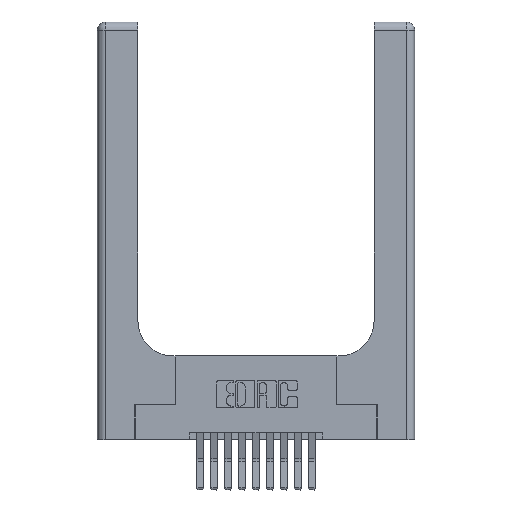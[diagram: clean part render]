
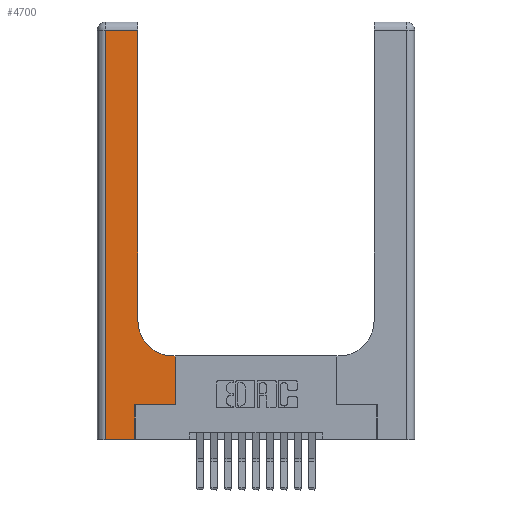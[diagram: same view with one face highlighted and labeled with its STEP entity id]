
A CAD part, top view. The second image highlights one B-rep face of the part: STEP entity #4700.
In plain terms, the highlighted planar face has unit normal (0, 0, 1).
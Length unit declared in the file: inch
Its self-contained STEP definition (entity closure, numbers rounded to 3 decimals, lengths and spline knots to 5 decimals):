
#72 = LINE ( 'NONE', #14565, #12407 ) ;
#222 = EDGE_CURVE ( 'NONE', #7299, #13981, #5925, .T. ) ;
#307 = DIRECTION ( 'NONE',  ( 0., -1., 0. ) ) ;
#822 = CARTESIAN_POINT ( 'NONE',  ( 0., 3., 0.37 ) ) ;
#990 = CARTESIAN_POINT ( 'NONE',  ( 0.5415, 0.85, 0.37 ) ) ;
#1524 = CARTESIAN_POINT ( 'NONE',  ( 0.2915, 3., 0.37 ) ) ;
#1644 = FACE_OUTER_BOUND ( 'NONE', #4326, .T. ) ;
#2067 = VECTOR ( 'NONE', #12881, 39.37008 ) ;
#2114 = DIRECTION ( 'NONE',  ( 0., 0., -1. ) ) ;
#2183 = DIRECTION ( 'NONE',  ( 1., 0., 0. ) ) ;
#2291 = VECTOR ( 'NONE', #4145, 39.37008 ) ;
#2648 = CARTESIAN_POINT ( 'NONE',  ( 0.269, 0.25, 0.37 ) ) ;
#3165 = VECTOR ( 'NONE', #307, 39.37008 ) ;
#3362 = DIRECTION ( 'NONE',  ( 0., 0., -1. ) ) ;
#3465 = EDGE_CURVE ( 'NONE', #14264, #10648, #11820, .T. ) ;
#3478 = PLANE ( 'NONE',  #10093 ) ;
#3799 = LINE ( 'NONE', #9825, #3165 ) ;
#3899 = LINE ( 'NONE', #6429, #2067 ) ;
#4033 = LINE ( 'NONE', #15352, #6666 ) ;
#4145 = DIRECTION ( 'NONE',  ( 0., 1., 0. ) ) ;
#4220 = CARTESIAN_POINT ( 'NONE',  ( 0.5415, 0.6, 0.37 ) ) ;
#4270 = CARTESIAN_POINT ( 'NONE',  ( 0.5585, 0.25, 0.37 ) ) ;
#4326 = EDGE_LOOP ( 'NONE', ( #11768, #13753, #9797, #5466, #5655, #13110, #4332, #12403, #4634 ) ) ;
#4332 = ORIENTED_EDGE ( 'NONE', *, *, #6078, .T. ) ;
#4634 = ORIENTED_EDGE ( 'NONE', *, *, #4713, .T. ) ;
#4700 = ADVANCED_FACE ( 'NONE', ( #1644 ), #3478, .F. ) ;
#4713 = EDGE_CURVE ( 'NONE', #5835, #7299, #9153, .T. ) ;
#4761 = VERTEX_POINT ( 'NONE', #6194 ) ;
#4928 = VERTEX_POINT ( 'NONE', #14402 ) ;
#5466 = ORIENTED_EDGE ( 'NONE', *, *, #7401, .T. ) ;
#5625 = LINE ( 'NONE', #4270, #6683 ) ;
#5655 = ORIENTED_EDGE ( 'NONE', *, *, #11003, .T. ) ;
#5835 = VERTEX_POINT ( 'NONE', #4220 ) ;
#5925 = LINE ( 'NONE', #1524, #2291 ) ;
#6078 = EDGE_CURVE ( 'NONE', #10648, #4761, #5625, .T. ) ;
#6194 = CARTESIAN_POINT ( 'NONE',  ( 0.5585, 0.6, 0.37 ) ) ;
#6277 = EDGE_CURVE ( 'NONE', #4761, #5835, #4033, .T. ) ;
#6429 = CARTESIAN_POINT ( 'NONE',  ( 0., 2.94, 0.37 ) ) ;
#6666 = VECTOR ( 'NONE', #11762, 39.37008 ) ;
#6683 = VECTOR ( 'NONE', #10739, 39.37008 ) ;
#7299 = VERTEX_POINT ( 'NONE', #11788 ) ;
#7401 = EDGE_CURVE ( 'NONE', #13030, #4928, #72, .T. ) ;
#7614 = LINE ( 'NONE', #12504, #13249 ) ;
#7795 = CARTESIAN_POINT ( 'NONE',  ( 0.06, 0., 0.37 ) ) ;
#8512 = CARTESIAN_POINT ( 'NONE',  ( 0.06, 2.94, 0.37 ) ) ;
#9153 = CIRCLE ( 'NONE', #11802, 0.25 ) ;
#9394 = VECTOR ( 'NONE', #14858, 39.37008 ) ;
#9561 = EDGE_CURVE ( 'NONE', #11232, #13030, #3799, .T. ) ;
#9797 = ORIENTED_EDGE ( 'NONE', *, *, #9561, .T. ) ;
#9825 = CARTESIAN_POINT ( 'NONE',  ( 0.06, 3., 0.37 ) ) ;
#10093 = AXIS2_PLACEMENT_3D ( 'NONE', #822, #3362, #15098 ) ;
#10648 = VERTEX_POINT ( 'NONE', #13576 ) ;
#10739 = DIRECTION ( 'NONE',  ( 0., 1., 0. ) ) ;
#10819 = CARTESIAN_POINT ( 'NONE',  ( 0.2915, 2.94, 0.37 ) ) ;
#11003 = EDGE_CURVE ( 'NONE', #4928, #14264, #7614, .T. ) ;
#11232 = VERTEX_POINT ( 'NONE', #8512 ) ;
#11762 = DIRECTION ( 'NONE',  ( -1., 0., 0. ) ) ;
#11768 = ORIENTED_EDGE ( 'NONE', *, *, #222, .T. ) ;
#11788 = CARTESIAN_POINT ( 'NONE',  ( 0.2915, 0.85, 0.37 ) ) ;
#11802 = AXIS2_PLACEMENT_3D ( 'NONE', #990, #2114, #2183 ) ;
#11820 = LINE ( 'NONE', #14799, #9394 ) ;
#12063 = DIRECTION ( 'NONE',  ( 1., 0., 0. ) ) ;
#12394 = DIRECTION ( 'NONE',  ( 0., 1., 0. ) ) ;
#12403 = ORIENTED_EDGE ( 'NONE', *, *, #6277, .T. ) ;
#12407 = VECTOR ( 'NONE', #12063, 39.37008 ) ;
#12504 = CARTESIAN_POINT ( 'NONE',  ( 0.269, 0., 0.37 ) ) ;
#12881 = DIRECTION ( 'NONE',  ( -1., 0., 0. ) ) ;
#13030 = VERTEX_POINT ( 'NONE', #7795 ) ;
#13110 = ORIENTED_EDGE ( 'NONE', *, *, #3465, .T. ) ;
#13249 = VECTOR ( 'NONE', #12394, 39.37008 ) ;
#13576 = CARTESIAN_POINT ( 'NONE',  ( 0.5585, 0.25, 0.37 ) ) ;
#13753 = ORIENTED_EDGE ( 'NONE', *, *, #15255, .T. ) ;
#13981 = VERTEX_POINT ( 'NONE', #10819 ) ;
#14264 = VERTEX_POINT ( 'NONE', #2648 ) ;
#14402 = CARTESIAN_POINT ( 'NONE',  ( 0.269, 0., 0.37 ) ) ;
#14565 = CARTESIAN_POINT ( 'NONE',  ( 0., 0., 0.37 ) ) ;
#14799 = CARTESIAN_POINT ( 'NONE',  ( 0.269, 0.25, 0.37 ) ) ;
#14858 = DIRECTION ( 'NONE',  ( 1., 0., 0. ) ) ;
#15098 = DIRECTION ( 'NONE',  ( -1., 0., 0. ) ) ;
#15255 = EDGE_CURVE ( 'NONE', #13981, #11232, #3899, .T. ) ;
#15352 = CARTESIAN_POINT ( 'NONE',  ( 0.2915, 0.6, 0.37 ) ) ;
